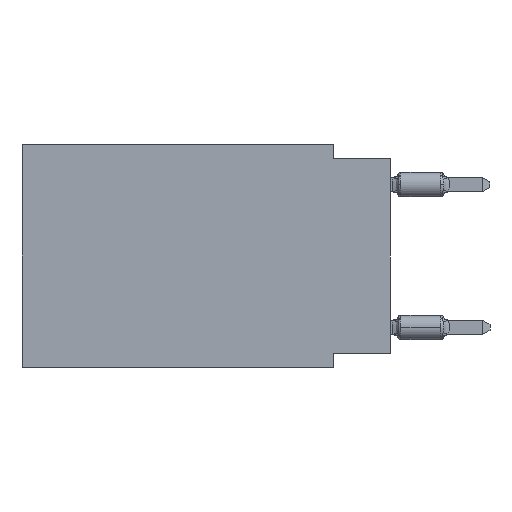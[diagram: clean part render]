
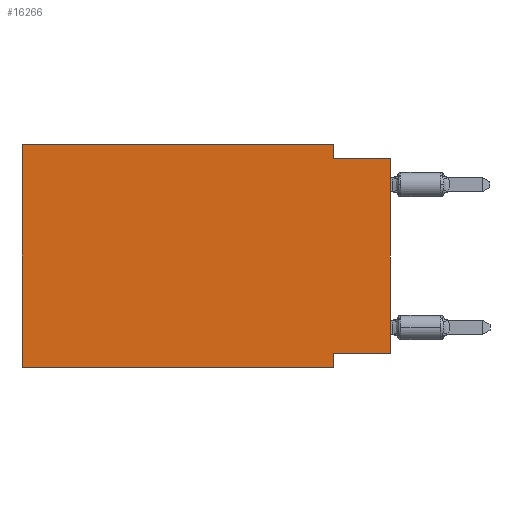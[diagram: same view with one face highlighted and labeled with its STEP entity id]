
A CAD part, left-side view. The second image highlights one B-rep face of the part: STEP entity #16266.
In plain terms, the highlighted planar face has unit normal (-1, 0, 0).
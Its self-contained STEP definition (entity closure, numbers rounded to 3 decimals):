
#155 = DIRECTION ( 'NONE',  ( 0., 0., -1. ) ) ;
#400 = VERTEX_POINT ( 'NONE', #9462 ) ;
#519 = ORIENTED_EDGE ( 'NONE', *, *, #1899, .F. ) ;
#1899 = EDGE_CURVE ( 'NONE', #7525, #8364, #7008, .T. ) ;
#1910 = ORIENTED_EDGE ( 'NONE', *, *, #15313, .T. ) ;
#2250 = ORIENTED_EDGE ( 'NONE', *, *, #20629, .F. ) ;
#2590 = VECTOR ( 'NONE', #3251, 1000. ) ;
#2710 = EDGE_LOOP ( 'NONE', ( #17621, #2250, #18248, #12842, #13373, #1910, #18699, #519 ) ) ;
#2750 = VECTOR ( 'NONE', #155, 1000. ) ;
#3251 = DIRECTION ( 'NONE',  ( 0., 0., 1. ) ) ;
#3761 = CARTESIAN_POINT ( 'NONE',  ( 0., 0., -9.271 ) ) ;
#4503 = DIRECTION ( 'NONE',  ( 1., 0., 0. ) ) ;
#4680 = VERTEX_POINT ( 'NONE', #5627 ) ;
#4820 = EDGE_CURVE ( 'NONE', #13176, #9971, #11141, .T. ) ;
#4877 = DIRECTION ( 'NONE',  ( 0., -1., 0. ) ) ;
#5082 = VERTEX_POINT ( 'NONE', #10272 ) ;
#5086 = DIRECTION ( 'NONE',  ( 0., 0., 1. ) ) ;
#5363 = DIRECTION ( 'NONE',  ( 0., -1., 0. ) ) ;
#5567 = VERTEX_POINT ( 'NONE', #13017 ) ;
#5620 = AXIS2_PLACEMENT_3D ( 'NONE', #19446, #4503, #9476 ) ;
#5627 = CARTESIAN_POINT ( 'NONE',  ( 0., 0., -0.635 ) ) ;
#5834 = VECTOR ( 'NONE', #18454, 1000. ) ;
#5926 = CARTESIAN_POINT ( 'NONE',  ( 0., 16.383, 0. ) ) ;
#6204 = EDGE_CURVE ( 'NONE', #7525, #4680, #20121, .T. ) ;
#7008 = LINE ( 'NONE', #3761, #19878 ) ;
#7094 = LINE ( 'NONE', #10128, #18840 ) ;
#7145 = VECTOR ( 'NONE', #4877, 1000. ) ;
#7525 = VERTEX_POINT ( 'NONE', #11873 ) ;
#7854 = FACE_OUTER_BOUND ( 'NONE', #2710, .T. ) ;
#8364 = VERTEX_POINT ( 'NONE', #9655 ) ;
#9462 = CARTESIAN_POINT ( 'NONE',  ( 0., 16.383, -9.906 ) ) ;
#9476 = DIRECTION ( 'NONE',  ( 0., 0., -1. ) ) ;
#9655 = CARTESIAN_POINT ( 'NONE',  ( 0., 2.54, -9.271 ) ) ;
#9943 = CARTESIAN_POINT ( 'NONE',  ( 0., 0., 0. ) ) ;
#9971 = VERTEX_POINT ( 'NONE', #19924 ) ;
#10128 = CARTESIAN_POINT ( 'NONE',  ( 0., 16.383, -9.906 ) ) ;
#10272 = CARTESIAN_POINT ( 'NONE',  ( 0., 2.54, -0.635 ) ) ;
#10655 = CARTESIAN_POINT ( 'NONE',  ( 0., 16.383, 0. ) ) ;
#11141 = LINE ( 'NONE', #5926, #15094 ) ;
#11462 = VECTOR ( 'NONE', #5086, 1000. ) ;
#11873 = CARTESIAN_POINT ( 'NONE',  ( 0., 0., -9.271 ) ) ;
#11942 = CARTESIAN_POINT ( 'NONE',  ( 0., 2.54, 0. ) ) ;
#12085 = EDGE_CURVE ( 'NONE', #400, #13176, #17881, .T. ) ;
#12842 = ORIENTED_EDGE ( 'NONE', *, *, #4820, .F. ) ;
#13017 = CARTESIAN_POINT ( 'NONE',  ( 0., 2.54, -9.906 ) ) ;
#13176 = VERTEX_POINT ( 'NONE', #10655 ) ;
#13351 = LINE ( 'NONE', #11942, #2750 ) ;
#13373 = ORIENTED_EDGE ( 'NONE', *, *, #12085, .F. ) ;
#13430 = LINE ( 'NONE', #18533, #7145 ) ;
#13455 = LINE ( 'NONE', #20059, #5834 ) ;
#14742 = CARTESIAN_POINT ( 'NONE',  ( 0., 16.383, 0. ) ) ;
#15094 = VECTOR ( 'NONE', #17760, 1000. ) ;
#15313 = EDGE_CURVE ( 'NONE', #400, #5567, #7094, .T. ) ;
#15365 = DIRECTION ( 'NONE',  ( 0., 1., 0. ) ) ;
#16266 = ADVANCED_FACE ( 'NONE', ( #7854 ), #20840, .F. ) ;
#17136 = EDGE_CURVE ( 'NONE', #8364, #5567, #13455, .T. ) ;
#17621 = ORIENTED_EDGE ( 'NONE', *, *, #6204, .T. ) ;
#17760 = DIRECTION ( 'NONE',  ( 0., -1., 0. ) ) ;
#17881 = LINE ( 'NONE', #14742, #11462 ) ;
#18248 = ORIENTED_EDGE ( 'NONE', *, *, #19094, .F. ) ;
#18454 = DIRECTION ( 'NONE',  ( 0., 0., -1. ) ) ;
#18533 = CARTESIAN_POINT ( 'NONE',  ( 0., 0., -0.635 ) ) ;
#18699 = ORIENTED_EDGE ( 'NONE', *, *, #17136, .F. ) ;
#18840 = VECTOR ( 'NONE', #5363, 1000. ) ;
#19094 = EDGE_CURVE ( 'NONE', #9971, #5082, #13351, .T. ) ;
#19446 = CARTESIAN_POINT ( 'NONE',  ( 0., 16.383, 0. ) ) ;
#19878 = VECTOR ( 'NONE', #15365, 1000. ) ;
#19924 = CARTESIAN_POINT ( 'NONE',  ( 0., 2.54, 0. ) ) ;
#20059 = CARTESIAN_POINT ( 'NONE',  ( 0., 2.54, -9.906 ) ) ;
#20121 = LINE ( 'NONE', #9943, #2590 ) ;
#20629 = EDGE_CURVE ( 'NONE', #5082, #4680, #13430, .T. ) ;
#20840 = PLANE ( 'NONE',  #5620 ) ;
